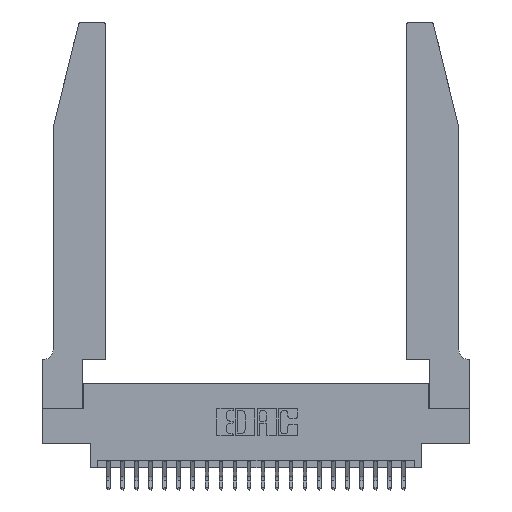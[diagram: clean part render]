
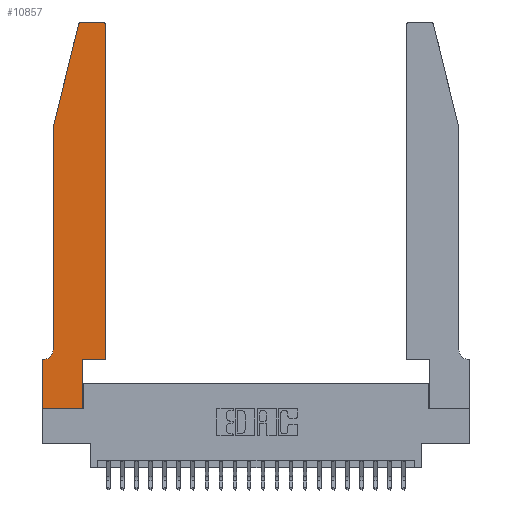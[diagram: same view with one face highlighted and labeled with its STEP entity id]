
A CAD part, top view. The second image highlights one B-rep face of the part: STEP entity #10857.
In plain terms, the highlighted planar face has unit normal (0, 0, 1).
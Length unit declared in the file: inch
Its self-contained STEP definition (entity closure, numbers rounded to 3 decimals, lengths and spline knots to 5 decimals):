
#136 = EDGE_CURVE ( 'NONE', #21838, #22428, #4636, .T. ) ;
#460 = DIRECTION ( 'NONE',  ( 0., 0., 1. ) ) ;
#517 = VECTOR ( 'NONE', #19617, 39.37008 ) ;
#1138 = LINE ( 'NONE', #17252, #11514 ) ;
#1208 = CARTESIAN_POINT ( 'NONE',  ( 0.25487, 2.72718, 0.37 ) ) ;
#1906 = EDGE_CURVE ( 'NONE', #20841, #13223, #6324, .T. ) ;
#1942 = VERTEX_POINT ( 'NONE', #13972 ) ;
#2602 = CARTESIAN_POINT ( 'NONE',  ( 0.4505, 0.35, 0.37 ) ) ;
#3103 = EDGE_CURVE ( 'NONE', #22428, #6923, #15421, .T. ) ;
#3166 = CARTESIAN_POINT ( 'NONE',  ( 0.0055, 0.42, 0.37 ) ) ;
#3362 = DIRECTION ( 'NONE',  ( 0., 1., 0. ) ) ;
#3720 = CARTESIAN_POINT ( 'NONE',  ( 0., 0.35, 0.37 ) ) ;
#3864 = VECTOR ( 'NONE', #11318, 39.37008 ) ;
#4096 = CARTESIAN_POINT ( 'NONE',  ( 0.4205, 2.75, 0.37 ) ) ;
#4320 = ORIENTED_EDGE ( 'NONE', *, *, #17610, .T. ) ;
#4412 = AXIS2_PLACEMENT_3D ( 'NONE', #8545, #22082, #10498 ) ;
#4465 = PLANE ( 'NONE',  #4867 ) ;
#4547 = VERTEX_POINT ( 'NONE', #1208 ) ;
#4636 = LINE ( 'NONE', #2602, #14342 ) ;
#4867 = AXIS2_PLACEMENT_3D ( 'NONE', #10246, #10326, #23814 ) ;
#5120 = DIRECTION ( 'NONE',  ( -1., 0., 0. ) ) ;
#5190 = ORIENTED_EDGE ( 'NONE', *, *, #136, .T. ) ;
#5300 = DIRECTION ( 'NONE',  ( 1., 0., 0. ) ) ;
#5589 = CARTESIAN_POINT ( 'NONE',  ( 0.2865, 0.35, 0.37 ) ) ;
#5613 = DIRECTION ( 'NONE',  ( -0.239, -0.971, 0. ) ) ;
#5977 = ORIENTED_EDGE ( 'NONE', *, *, #13419, .T. ) ;
#6145 = VECTOR ( 'NONE', #19554, 39.37008 ) ;
#6324 = LINE ( 'NONE', #17683, #517 ) ;
#6923 = VERTEX_POINT ( 'NONE', #4096 ) ;
#7105 = DIRECTION ( 'NONE',  ( -1., 0., 0. ) ) ;
#7603 = CARTESIAN_POINT ( 'NONE',  ( 0.0755, 0.42, 0.37 ) ) ;
#7739 = EDGE_CURVE ( 'NONE', #18115, #21838, #17056, .T. ) ;
#7959 = CARTESIAN_POINT ( 'NONE',  ( 0.0755, 0.35, 0.37 ) ) ;
#8012 = CARTESIAN_POINT ( 'NONE',  ( 0.0755, 2., 0.37 ) ) ;
#8076 = ORIENTED_EDGE ( 'NONE', *, *, #3103, .T. ) ;
#8316 = VERTEX_POINT ( 'NONE', #19792 ) ;
#8545 = CARTESIAN_POINT ( 'NONE',  ( 0.284, 2.72, 0.37 ) ) ;
#8709 = EDGE_CURVE ( 'NONE', #13223, #18288, #19693, .T. ) ;
#9038 = LINE ( 'NONE', #24778, #3864 ) ;
#9528 = VECTOR ( 'NONE', #14845, 39.37008 ) ;
#9937 = FACE_OUTER_BOUND ( 'NONE', #13612, .T. ) ;
#10246 = CARTESIAN_POINT ( 'NONE',  ( 0., 0.35, 0.37 ) ) ;
#10326 = DIRECTION ( 'NONE',  ( 0., 0., 1. ) ) ;
#10498 = DIRECTION ( 'NONE',  ( 1., 0., 0. ) ) ;
#10624 = CIRCLE ( 'NONE', #4412, 0.03 ) ;
#10857 = ADVANCED_FACE ( 'NONE', ( #9937 ), #4465, .T. ) ;
#11079 = ORIENTED_EDGE ( 'NONE', *, *, #7739, .T. ) ;
#11318 = DIRECTION ( 'NONE',  ( 0., 1., 0. ) ) ;
#11514 = VECTOR ( 'NONE', #5613, 39.37008 ) ;
#12139 = ORIENTED_EDGE ( 'NONE', *, *, #21141, .T. ) ;
#12153 = CARTESIAN_POINT ( 'NONE',  ( 0.4205, 2.72, 0.37 ) ) ;
#12907 = CARTESIAN_POINT ( 'NONE',  ( 0.0755, 2., 0.37 ) ) ;
#13223 = VERTEX_POINT ( 'NONE', #19065 ) ;
#13386 = AXIS2_PLACEMENT_3D ( 'NONE', #12153, #460, #14075 ) ;
#13419 = EDGE_CURVE ( 'NONE', #1942, #20841, #21598, .T. ) ;
#13612 = EDGE_LOOP ( 'NONE', ( #22650, #12139, #15028, #17671, #19182, #5977, #16439, #22054, #4320, #11079, #5190, #8076 ) ) ;
#13751 = CARTESIAN_POINT ( 'NONE',  ( 0.4505, 2.72, 0.37 ) ) ;
#13972 = CARTESIAN_POINT ( 'NONE',  ( 0.0055, 0.35, 0.37 ) ) ;
#14075 = DIRECTION ( 'NONE',  ( 1., 0., 0. ) ) ;
#14342 = VECTOR ( 'NONE', #3362, 39.37008 ) ;
#14379 = EDGE_CURVE ( 'NONE', #22960, #1942, #18872, .T. ) ;
#14515 = VECTOR ( 'NONE', #7105, 39.37008 ) ;
#14540 = VECTOR ( 'NONE', #5300, 39.37008 ) ;
#14845 = DIRECTION ( 'NONE',  ( 0., -1., 0. ) ) ;
#15028 = ORIENTED_EDGE ( 'NONE', *, *, #21811, .T. ) ;
#15421 = CIRCLE ( 'NONE', #13386, 0.03 ) ;
#15950 = CARTESIAN_POINT ( 'NONE',  ( 0.2865, 0., 0.37 ) ) ;
#16439 = ORIENTED_EDGE ( 'NONE', *, *, #1906, .T. ) ;
#16443 = VECTOR ( 'NONE', #20146, 39.37008 ) ;
#16760 = DIRECTION ( 'NONE',  ( 0., 0., -1. ) ) ;
#16885 = EDGE_CURVE ( 'NONE', #6923, #8316, #24169, .T. ) ;
#17056 = LINE ( 'NONE', #18209, #16443 ) ;
#17204 = VERTEX_POINT ( 'NONE', #8012 ) ;
#17252 = CARTESIAN_POINT ( 'NONE',  ( 0.0755, 2., 0.37 ) ) ;
#17610 = EDGE_CURVE ( 'NONE', #18288, #18115, #9038, .T. ) ;
#17671 = ORIENTED_EDGE ( 'NONE', *, *, #20637, .T. ) ;
#17683 = CARTESIAN_POINT ( 'NONE',  ( 0., 0., 0.37 ) ) ;
#18115 = VERTEX_POINT ( 'NONE', #5589 ) ;
#18209 = CARTESIAN_POINT ( 'NONE',  ( 0.4505, 0.35, 0.37 ) ) ;
#18288 = VERTEX_POINT ( 'NONE', #15950 ) ;
#18841 = CARTESIAN_POINT ( 'NONE',  ( 0., 0., 0.37 ) ) ;
#18872 = CIRCLE ( 'NONE', #19256, 0.07 ) ;
#19065 = CARTESIAN_POINT ( 'NONE',  ( 0., 0., 0.37 ) ) ;
#19182 = ORIENTED_EDGE ( 'NONE', *, *, #14379, .T. ) ;
#19256 = AXIS2_PLACEMENT_3D ( 'NONE', #3166, #16760, #5120 ) ;
#19554 = DIRECTION ( 'NONE',  ( -1., 0., 0. ) ) ;
#19617 = DIRECTION ( 'NONE',  ( 0., -1., 0. ) ) ;
#19693 = LINE ( 'NONE', #18841, #14540 ) ;
#19792 = CARTESIAN_POINT ( 'NONE',  ( 0.284, 2.75, 0.37 ) ) ;
#19812 = LINE ( 'NONE', #12907, #9528 ) ;
#20146 = DIRECTION ( 'NONE',  ( 1., 0., 0. ) ) ;
#20635 = CARTESIAN_POINT ( 'NONE',  ( 0.2605, 2.75, 0.37 ) ) ;
#20637 = EDGE_CURVE ( 'NONE', #17204, #22960, #19812, .T. ) ;
#20841 = VERTEX_POINT ( 'NONE', #3720 ) ;
#21141 = EDGE_CURVE ( 'NONE', #8316, #4547, #10624, .T. ) ;
#21598 = LINE ( 'NONE', #7959, #6145 ) ;
#21811 = EDGE_CURVE ( 'NONE', #4547, #17204, #1138, .T. ) ;
#21838 = VERTEX_POINT ( 'NONE', #24940 ) ;
#22054 = ORIENTED_EDGE ( 'NONE', *, *, #8709, .T. ) ;
#22082 = DIRECTION ( 'NONE',  ( 0., 0., 1. ) ) ;
#22428 = VERTEX_POINT ( 'NONE', #13751 ) ;
#22650 = ORIENTED_EDGE ( 'NONE', *, *, #16885, .T. ) ;
#22960 = VERTEX_POINT ( 'NONE', #7603 ) ;
#23814 = DIRECTION ( 'NONE',  ( 1., 0., 0. ) ) ;
#24169 = LINE ( 'NONE', #20635, #14515 ) ;
#24778 = CARTESIAN_POINT ( 'NONE',  ( 0.2865, 0.35, 0.37 ) ) ;
#24940 = CARTESIAN_POINT ( 'NONE',  ( 0.4505, 0.35, 0.37 ) ) ;
